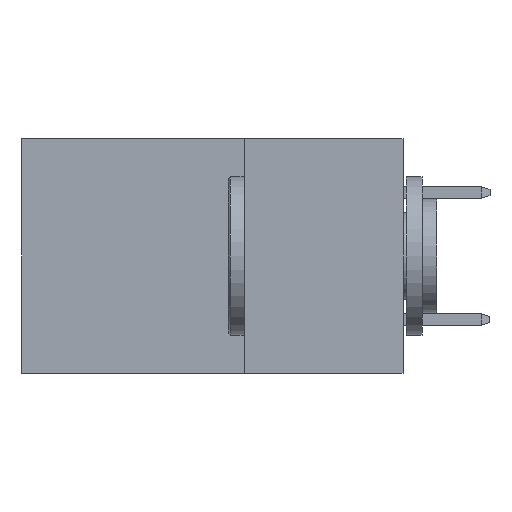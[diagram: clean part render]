
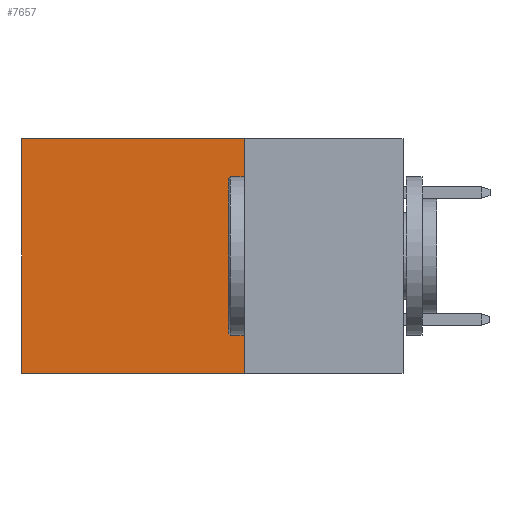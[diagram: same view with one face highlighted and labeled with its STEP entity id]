
A CAD part, left-side view. The second image highlights one B-rep face of the part: STEP entity #7657.
In plain terms, the highlighted planar face has unit normal (-1, 0, 0).
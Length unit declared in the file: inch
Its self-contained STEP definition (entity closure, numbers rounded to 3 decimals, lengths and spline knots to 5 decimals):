
#127 = ORIENTED_EDGE ( 'NONE', *, *, #7225, .F. ) ;
#386 = ORIENTED_EDGE ( 'NONE', *, *, #11494, .T. ) ;
#805 = CARTESIAN_POINT ( 'NONE',  ( 0.2875, 0.25, 0. ) ) ;
#945 = LINE ( 'NONE', #10858, #9581 ) ;
#1573 = CARTESIAN_POINT ( 'NONE',  ( 0.2875, 0.25, -0.37 ) ) ;
#1739 = CARTESIAN_POINT ( 'NONE',  ( 0.2875, 0.6, 0. ) ) ;
#1811 = LINE ( 'NONE', #1739, #4069 ) ;
#1933 = EDGE_CURVE ( 'NONE', #8900, #2242, #945, .T. ) ;
#2242 = VERTEX_POINT ( 'NONE', #1573 ) ;
#2482 = DIRECTION ( 'NONE',  ( 0., 1., 0. ) ) ;
#2748 = VERTEX_POINT ( 'NONE', #12203 ) ;
#3984 = DIRECTION ( 'NONE',  ( 1., 0., 0. ) ) ;
#4069 = VECTOR ( 'NONE', #4800, 39.37008 ) ;
#4511 = CARTESIAN_POINT ( 'NONE',  ( 0.2875, 0.25, 0. ) ) ;
#4784 = ORIENTED_EDGE ( 'NONE', *, *, #1933, .F. ) ;
#4800 = DIRECTION ( 'NONE',  ( 0., 0., -1. ) ) ;
#5547 = VERTEX_POINT ( 'NONE', #11239 ) ;
#6016 = LINE ( 'NONE', #8059, #10903 ) ;
#6993 = FACE_OUTER_BOUND ( 'NONE', #10486, .T. ) ;
#7225 = EDGE_CURVE ( 'NONE', #2242, #5547, #6016, .T. ) ;
#7657 = ADVANCED_FACE ( 'NONE', ( #6993 ), #7915, .F. ) ;
#7915 = PLANE ( 'NONE',  #9874 ) ;
#7942 = VECTOR ( 'NONE', #2482, 39.37008 ) ;
#8059 = CARTESIAN_POINT ( 'NONE',  ( 0.2875, 0.25, -0.37 ) ) ;
#8900 = VERTEX_POINT ( 'NONE', #9308 ) ;
#9308 = CARTESIAN_POINT ( 'NONE',  ( 0.2875, 0.25, 0. ) ) ;
#9474 = ORIENTED_EDGE ( 'NONE', *, *, #12497, .T. ) ;
#9581 = VECTOR ( 'NONE', #10006, 39.37008 ) ;
#9874 = AXIS2_PLACEMENT_3D ( 'NONE', #805, #3984, #10982 ) ;
#10006 = DIRECTION ( 'NONE',  ( 0., 0., -1. ) ) ;
#10486 = EDGE_LOOP ( 'NONE', ( #9474, #127, #4784, #386 ) ) ;
#10858 = CARTESIAN_POINT ( 'NONE',  ( 0.2875, 0.25, 0. ) ) ;
#10903 = VECTOR ( 'NONE', #11848, 39.37008 ) ;
#10982 = DIRECTION ( 'NONE',  ( 0., 0., -1. ) ) ;
#11239 = CARTESIAN_POINT ( 'NONE',  ( 0.2875, 0.6, -0.37 ) ) ;
#11430 = LINE ( 'NONE', #4511, #7942 ) ;
#11494 = EDGE_CURVE ( 'NONE', #8900, #2748, #11430, .T. ) ;
#11848 = DIRECTION ( 'NONE',  ( 0., 1., 0. ) ) ;
#12203 = CARTESIAN_POINT ( 'NONE',  ( 0.2875, 0.6, 0. ) ) ;
#12497 = EDGE_CURVE ( 'NONE', #2748, #5547, #1811, .T. ) ;
